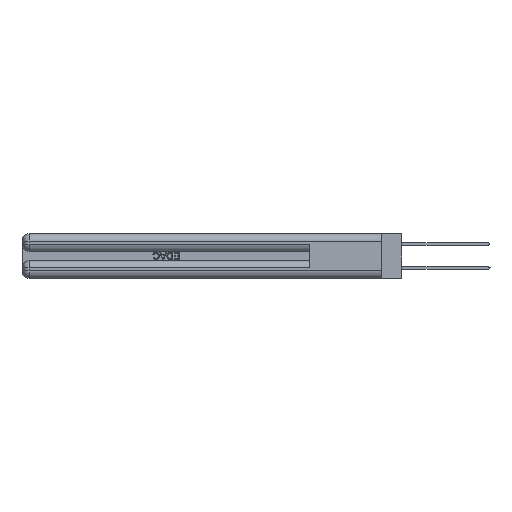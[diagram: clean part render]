
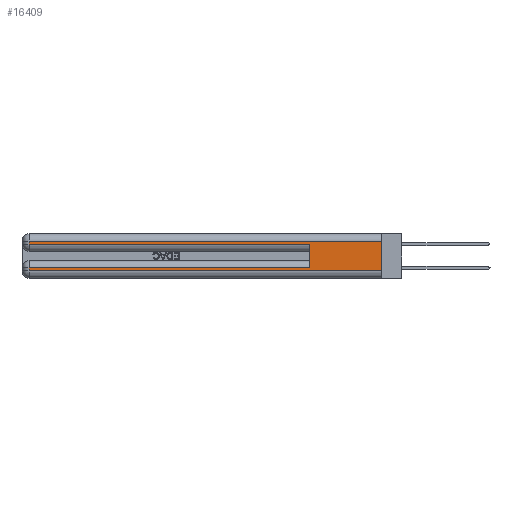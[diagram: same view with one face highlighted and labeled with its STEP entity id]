
A CAD part, left-side view. The second image highlights one B-rep face of the part: STEP entity #16409.
In plain terms, the highlighted planar face has unit normal (-1, 0, 0).
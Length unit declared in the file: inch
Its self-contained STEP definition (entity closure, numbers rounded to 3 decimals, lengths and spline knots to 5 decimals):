
#311 = VERTEX_POINT ( 'NONE', #25168 ) ;
#744 = EDGE_CURVE ( 'NONE', #26968, #311, #22765, .T. ) ;
#1198 = EDGE_CURVE ( 'NONE', #31497, #3415, #33818, .T. ) ;
#1275 = LINE ( 'NONE', #4933, #23317 ) ;
#2162 = EDGE_CURVE ( 'NONE', #34960, #17774, #32582, .T. ) ;
#2203 = ORIENTED_EDGE ( 'NONE', *, *, #3909, .T. ) ;
#3415 = VERTEX_POINT ( 'NONE', #20408 ) ;
#3909 = EDGE_CURVE ( 'NONE', #30333, #17774, #34945, .T. ) ;
#4024 = ORIENTED_EDGE ( 'NONE', *, *, #33705, .T. ) ;
#4040 = EDGE_CURVE ( 'NONE', #31497, #31704, #21833, .T. ) ;
#4515 = DIRECTION ( 'NONE',  ( 0., 1., 0. ) ) ;
#4933 = CARTESIAN_POINT ( 'NONE',  ( 0., 0., 0.31 ) ) ;
#5100 = CARTESIAN_POINT ( 'NONE',  ( 0., 0., 0.31 ) ) ;
#6180 = LINE ( 'NONE', #24668, #21210 ) ;
#7228 = CARTESIAN_POINT ( 'NONE',  ( 0., 0., 0.06 ) ) ;
#7345 = AXIS2_PLACEMENT_3D ( 'NONE', #29581, #13604, #10462 ) ;
#8599 = ORIENTED_EDGE ( 'NONE', *, *, #1198, .F. ) ;
#8883 = EDGE_LOOP ( 'NONE', ( #34940, #28514, #10416, #4024, #8599, #37660, #35231, #2203 ) ) ;
#9099 = DIRECTION ( 'NONE',  ( 0., -1., 0. ) ) ;
#10416 = ORIENTED_EDGE ( 'NONE', *, *, #744, .T. ) ;
#10462 = DIRECTION ( 'NONE',  ( 0., 0., -1. ) ) ;
#11167 = CARTESIAN_POINT ( 'NONE',  ( 0., 2.94, 0.31 ) ) ;
#11396 = LINE ( 'NONE', #31374, #23390 ) ;
#13491 = DIRECTION ( 'NONE',  ( 0., 0., -1. ) ) ;
#13604 = DIRECTION ( 'NONE',  ( 1., 0., 0. ) ) ;
#14488 = EDGE_CURVE ( 'NONE', #31704, #30333, #11396, .T. ) ;
#16409 = ADVANCED_FACE ( 'NONE', ( #20307 ), #33242, .F. ) ;
#16845 = DIRECTION ( 'NONE',  ( 0., 0., 1. ) ) ;
#17774 = VERTEX_POINT ( 'NONE', #7228 ) ;
#18717 = DIRECTION ( 'NONE',  ( 0., 0., -1. ) ) ;
#18806 = CARTESIAN_POINT ( 'NONE',  ( 0., 0.6, 0.085 ) ) ;
#20307 = FACE_OUTER_BOUND ( 'NONE', #8883, .T. ) ;
#20408 = CARTESIAN_POINT ( 'NONE',  ( 0., 0.6, 0.285 ) ) ;
#21210 = VECTOR ( 'NONE', #9099, 39.37008 ) ;
#21665 = DIRECTION ( 'NONE',  ( 0., 0., -1. ) ) ;
#21833 = LINE ( 'NONE', #30164, #37418 ) ;
#21850 = DIRECTION ( 'NONE',  ( 0., 1., 0. ) ) ;
#22299 = VECTOR ( 'NONE', #13491, 39.37008 ) ;
#22309 = VECTOR ( 'NONE', #35770, 39.37008 ) ;
#22765 = LINE ( 'NONE', #39413, #22299 ) ;
#23317 = VECTOR ( 'NONE', #4515, 39.37008 ) ;
#23390 = VECTOR ( 'NONE', #21665, 39.37008 ) ;
#24133 = CARTESIAN_POINT ( 'NONE',  ( 0., 0., 0.06 ) ) ;
#24668 = CARTESIAN_POINT ( 'NONE',  ( 0., 0., 0.285 ) ) ;
#25168 = CARTESIAN_POINT ( 'NONE',  ( 0., 2.94, 0.285 ) ) ;
#26968 = VERTEX_POINT ( 'NONE', #11167 ) ;
#28264 = CARTESIAN_POINT ( 'NONE',  ( 0., 0., 0.37 ) ) ;
#28514 = ORIENTED_EDGE ( 'NONE', *, *, #36850, .T. ) ;
#29581 = CARTESIAN_POINT ( 'NONE',  ( 0., 0., 0.37 ) ) ;
#30164 = CARTESIAN_POINT ( 'NONE',  ( 0., 0., 0.085 ) ) ;
#30333 = VERTEX_POINT ( 'NONE', #33179 ) ;
#31374 = CARTESIAN_POINT ( 'NONE',  ( 0., 2.94, 0.37 ) ) ;
#31497 = VERTEX_POINT ( 'NONE', #18806 ) ;
#31704 = VERTEX_POINT ( 'NONE', #37173 ) ;
#32582 = LINE ( 'NONE', #28264, #36602 ) ;
#32853 = CARTESIAN_POINT ( 'NONE',  ( 0., 0.6, 0.145 ) ) ;
#33179 = CARTESIAN_POINT ( 'NONE',  ( 0., 2.94, 0.06 ) ) ;
#33242 = PLANE ( 'NONE',  #7345 ) ;
#33705 = EDGE_CURVE ( 'NONE', #311, #3415, #6180, .T. ) ;
#33818 = LINE ( 'NONE', #32853, #34867 ) ;
#34867 = VECTOR ( 'NONE', #16845, 39.37008 ) ;
#34940 = ORIENTED_EDGE ( 'NONE', *, *, #2162, .F. ) ;
#34945 = LINE ( 'NONE', #24133, #22309 ) ;
#34960 = VERTEX_POINT ( 'NONE', #5100 ) ;
#35231 = ORIENTED_EDGE ( 'NONE', *, *, #14488, .T. ) ;
#35770 = DIRECTION ( 'NONE',  ( 0., -1., 0. ) ) ;
#36602 = VECTOR ( 'NONE', #18717, 39.37008 ) ;
#36850 = EDGE_CURVE ( 'NONE', #34960, #26968, #1275, .T. ) ;
#37173 = CARTESIAN_POINT ( 'NONE',  ( 0., 2.94, 0.085 ) ) ;
#37418 = VECTOR ( 'NONE', #21850, 39.37008 ) ;
#37660 = ORIENTED_EDGE ( 'NONE', *, *, #4040, .T. ) ;
#39413 = CARTESIAN_POINT ( 'NONE',  ( 0., 2.94, 0.37 ) ) ;
